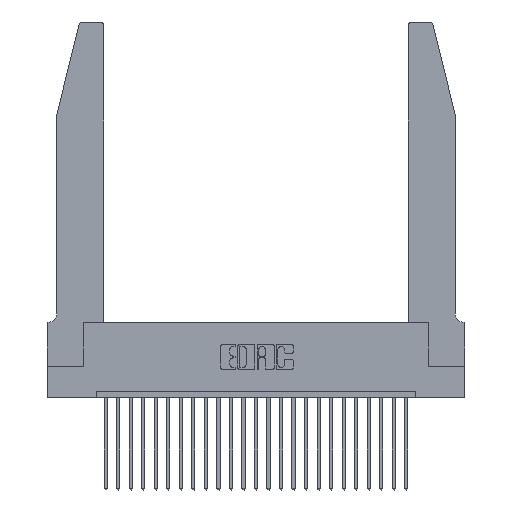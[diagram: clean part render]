
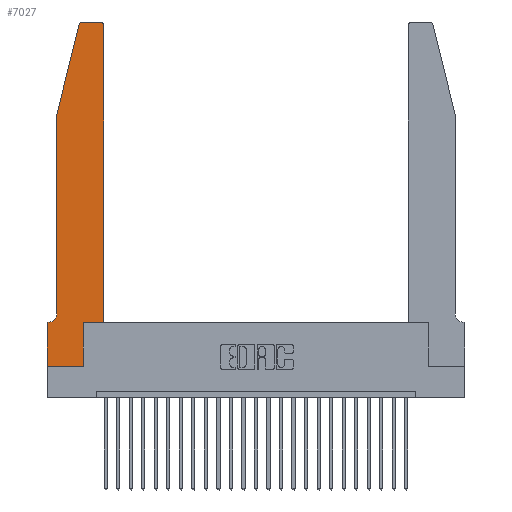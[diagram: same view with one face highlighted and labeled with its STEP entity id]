
A CAD part, top view. The second image highlights one B-rep face of the part: STEP entity #7027.
In plain terms, the highlighted planar face has unit normal (0, 0, 1).
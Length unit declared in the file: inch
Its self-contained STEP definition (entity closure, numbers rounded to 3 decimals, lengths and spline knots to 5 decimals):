
#467 = VECTOR ( 'NONE', #2612, 39.37008 ) ;
#808 = LINE ( 'NONE', #22629, #14178 ) ;
#1189 = DIRECTION ( 'NONE',  ( 0., -1., 0. ) ) ;
#1345 = LINE ( 'NONE', #20337, #15058 ) ;
#1466 = EDGE_CURVE ( 'NONE', #11984, #9487, #9271, .T. ) ;
#1625 = DIRECTION ( 'NONE',  ( -1., 0., 0. ) ) ;
#1629 = VERTEX_POINT ( 'NONE', #2782 ) ;
#2612 = DIRECTION ( 'NONE',  ( 1., 0., 0. ) ) ;
#2782 = CARTESIAN_POINT ( 'NONE',  ( 0.0055, 0.35, 0.37 ) ) ;
#3078 = DIRECTION ( 'NONE',  ( 0., -1., 0. ) ) ;
#3766 = CARTESIAN_POINT ( 'NONE',  ( 0.284, 2.75, 0.37 ) ) ;
#4122 = VERTEX_POINT ( 'NONE', #21520 ) ;
#5035 = EDGE_CURVE ( 'NONE', #19205, #18652, #22759, .T. ) ;
#5182 = CARTESIAN_POINT ( 'NONE',  ( 0.2865, 0.35, 0.37 ) ) ;
#5387 = CARTESIAN_POINT ( 'NONE',  ( 0.0755, 2., 0.37 ) ) ;
#5453 = EDGE_CURVE ( 'NONE', #11370, #20958, #14613, .T. ) ;
#5558 = VECTOR ( 'NONE', #1189, 39.37008 ) ;
#5580 = CARTESIAN_POINT ( 'NONE',  ( 0.0055, 0.42, 0.37 ) ) ;
#5592 = VECTOR ( 'NONE', #11091, 39.37008 ) ;
#6290 = CARTESIAN_POINT ( 'NONE',  ( 0.4505, 0.35, 0.37 ) ) ;
#6442 = PLANE ( 'NONE',  #8389 ) ;
#6463 = EDGE_CURVE ( 'NONE', #20958, #1629, #16738, .T. ) ;
#7027 = ADVANCED_FACE ( 'NONE', ( #21668 ), #6442, .T. ) ;
#7073 = DIRECTION ( 'NONE',  ( 0., 0., 1. ) ) ;
#7078 = EDGE_CURVE ( 'NONE', #19107, #11984, #808, .T. ) ;
#7686 = CARTESIAN_POINT ( 'NONE',  ( 0.0755, 0.35, 0.37 ) ) ;
#7689 = ORIENTED_EDGE ( 'NONE', *, *, #5035, .T. ) ;
#7800 = VERTEX_POINT ( 'NONE', #22589 ) ;
#7998 = EDGE_CURVE ( 'NONE', #1629, #19107, #25723, .T. ) ;
#8389 = AXIS2_PLACEMENT_3D ( 'NONE', #20246, #22357, #12406 ) ;
#8478 = ORIENTED_EDGE ( 'NONE', *, *, #7998, .T. ) ;
#8773 = EDGE_CURVE ( 'NONE', #10015, #7800, #1345, .T. ) ;
#9117 = ORIENTED_EDGE ( 'NONE', *, *, #10632, .T. ) ;
#9271 = LINE ( 'NONE', #22870, #467 ) ;
#9487 = VERTEX_POINT ( 'NONE', #25310 ) ;
#9568 = VERTEX_POINT ( 'NONE', #21334 ) ;
#9622 = EDGE_CURVE ( 'NONE', #18652, #11370, #23763, .T. ) ;
#9780 = ORIENTED_EDGE ( 'NONE', *, *, #5453, .T. ) ;
#10015 = VERTEX_POINT ( 'NONE', #23134 ) ;
#10632 = EDGE_CURVE ( 'NONE', #7800, #4122, #18657, .T. ) ;
#10825 = CARTESIAN_POINT ( 'NONE',  ( 0., 0.35, 0.37 ) ) ;
#10899 = DIRECTION ( 'NONE',  ( 1., 0., 0. ) ) ;
#10916 = ORIENTED_EDGE ( 'NONE', *, *, #1466, .T. ) ;
#11091 = DIRECTION ( 'NONE',  ( 0., 1., 0. ) ) ;
#11370 = VERTEX_POINT ( 'NONE', #24426 ) ;
#11454 = VECTOR ( 'NONE', #11928, 39.37008 ) ;
#11928 = DIRECTION ( 'NONE',  ( -1., 0., 0. ) ) ;
#11984 = VERTEX_POINT ( 'NONE', #20467 ) ;
#12127 = ORIENTED_EDGE ( 'NONE', *, *, #21831, .T. ) ;
#12384 = ORIENTED_EDGE ( 'NONE', *, *, #15934, .T. ) ;
#12406 = DIRECTION ( 'NONE',  ( 1., 0., 0. ) ) ;
#13728 = DIRECTION ( 'NONE',  ( -1., 0., 0. ) ) ;
#14178 = VECTOR ( 'NONE', #3078, 39.37008 ) ;
#14613 = LINE ( 'NONE', #5387, #5558 ) ;
#15058 = VECTOR ( 'NONE', #22624, 39.37008 ) ;
#15164 = DIRECTION ( 'NONE',  ( 1., 0., 0. ) ) ;
#15478 = LINE ( 'NONE', #19751, #11454 ) ;
#15589 = DIRECTION ( 'NONE',  ( 0., 0., 1. ) ) ;
#15934 = EDGE_CURVE ( 'NONE', #9487, #10015, #21604, .T. ) ;
#16738 = CIRCLE ( 'NONE', #24399, 0.07 ) ;
#16974 = CARTESIAN_POINT ( 'NONE',  ( 0.284, 2.72, 0.37 ) ) ;
#17062 = ORIENTED_EDGE ( 'NONE', *, *, #7078, .T. ) ;
#17156 = ORIENTED_EDGE ( 'NONE', *, *, #20081, .T. ) ;
#17406 = CARTESIAN_POINT ( 'NONE',  ( 0.0755, 2., 0.37 ) ) ;
#17504 = CARTESIAN_POINT ( 'NONE',  ( 0.0755, 0.42, 0.37 ) ) ;
#18084 = ORIENTED_EDGE ( 'NONE', *, *, #9622, .T. ) ;
#18417 = VECTOR ( 'NONE', #25390, 39.37008 ) ;
#18526 = VECTOR ( 'NONE', #19089, 39.37008 ) ;
#18652 = VERTEX_POINT ( 'NONE', #22933 ) ;
#18657 = LINE ( 'NONE', #6290, #5592 ) ;
#19071 = CIRCLE ( 'NONE', #23208, 0.03 ) ;
#19089 = DIRECTION ( 'NONE',  ( 0., 1., 0. ) ) ;
#19107 = VERTEX_POINT ( 'NONE', #10825 ) ;
#19161 = DIRECTION ( 'NONE',  ( 0., 0., -1. ) ) ;
#19205 = VERTEX_POINT ( 'NONE', #3766 ) ;
#19434 = VECTOR ( 'NONE', #1625, 39.37008 ) ;
#19751 = CARTESIAN_POINT ( 'NONE',  ( 0.2605, 2.75, 0.37 ) ) ;
#20081 = EDGE_CURVE ( 'NONE', #9568, #19205, #15478, .T. ) ;
#20246 = CARTESIAN_POINT ( 'NONE',  ( 0., 0.35, 0.37 ) ) ;
#20337 = CARTESIAN_POINT ( 'NONE',  ( 0.4505, 0.35, 0.37 ) ) ;
#20467 = CARTESIAN_POINT ( 'NONE',  ( 0., 0., 0.37 ) ) ;
#20904 = CARTESIAN_POINT ( 'NONE',  ( 0.4205, 2.72, 0.37 ) ) ;
#20958 = VERTEX_POINT ( 'NONE', #17504 ) ;
#21235 = ORIENTED_EDGE ( 'NONE', *, *, #8773, .T. ) ;
#21334 = CARTESIAN_POINT ( 'NONE',  ( 0.4205, 2.75, 0.37 ) ) ;
#21470 = ORIENTED_EDGE ( 'NONE', *, *, #6463, .T. ) ;
#21520 = CARTESIAN_POINT ( 'NONE',  ( 0.4505, 2.72, 0.37 ) ) ;
#21604 = LINE ( 'NONE', #5182, #18526 ) ;
#21668 = FACE_OUTER_BOUND ( 'NONE', #25399, .T. ) ;
#21831 = EDGE_CURVE ( 'NONE', #4122, #9568, #19071, .T. ) ;
#22357 = DIRECTION ( 'NONE',  ( 0., 0., 1. ) ) ;
#22589 = CARTESIAN_POINT ( 'NONE',  ( 0.4505, 0.35, 0.37 ) ) ;
#22624 = DIRECTION ( 'NONE',  ( 1., 0., 0. ) ) ;
#22629 = CARTESIAN_POINT ( 'NONE',  ( 0., 0., 0.37 ) ) ;
#22759 = CIRCLE ( 'NONE', #24717, 0.03 ) ;
#22870 = CARTESIAN_POINT ( 'NONE',  ( 0., 0., 0.37 ) ) ;
#22933 = CARTESIAN_POINT ( 'NONE',  ( 0.25487, 2.72718, 0.37 ) ) ;
#23134 = CARTESIAN_POINT ( 'NONE',  ( 0.2865, 0.35, 0.37 ) ) ;
#23208 = AXIS2_PLACEMENT_3D ( 'NONE', #20904, #15589, #10899 ) ;
#23763 = LINE ( 'NONE', #17406, #18417 ) ;
#24399 = AXIS2_PLACEMENT_3D ( 'NONE', #5580, #19161, #13728 ) ;
#24426 = CARTESIAN_POINT ( 'NONE',  ( 0.0755, 2., 0.37 ) ) ;
#24717 = AXIS2_PLACEMENT_3D ( 'NONE', #16974, #7073, #15164 ) ;
#25310 = CARTESIAN_POINT ( 'NONE',  ( 0.2865, 0., 0.37 ) ) ;
#25390 = DIRECTION ( 'NONE',  ( -0.239, -0.971, 0. ) ) ;
#25399 = EDGE_LOOP ( 'NONE', ( #17156, #7689, #18084, #9780, #21470, #8478, #17062, #10916, #12384, #21235, #9117, #12127 ) ) ;
#25723 = LINE ( 'NONE', #7686, #19434 ) ;
